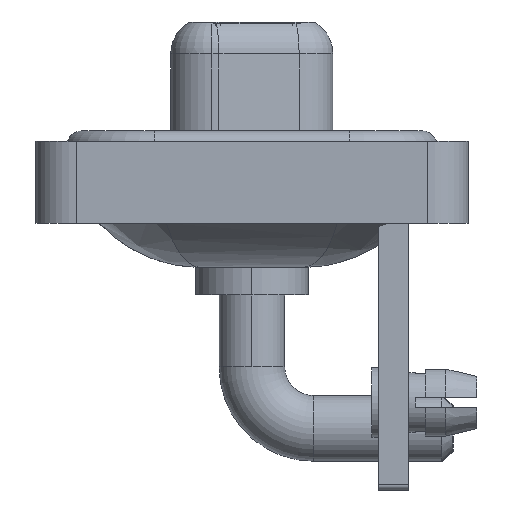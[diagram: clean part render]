
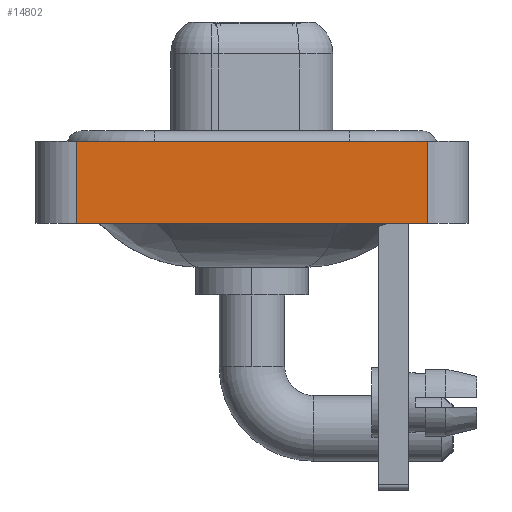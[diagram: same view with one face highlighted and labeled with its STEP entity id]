
A CAD part, left-side view. The second image highlights one B-rep face of the part: STEP entity #14802.
In plain terms, the highlighted planar face has unit normal (-1, 0, 0).
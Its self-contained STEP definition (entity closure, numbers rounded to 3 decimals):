
#95 = DIRECTION ( 'NONE',  ( 0., 0., 1. ) ) ;
#458 = ORIENTED_EDGE ( 'NONE', *, *, #13184, .T. ) ;
#964 = LINE ( 'NONE', #9850, #15194 ) ;
#982 = CARTESIAN_POINT ( 'NONE',  ( -7.25, 8.55, -3.6 ) ) ;
#1660 = CARTESIAN_POINT ( 'NONE',  ( -7.25, -8.55, -3.6 ) ) ;
#2927 = CARTESIAN_POINT ( 'NONE',  ( -7.25, -8.55, -3.6 ) ) ;
#3573 = LINE ( 'NONE', #8359, #3773 ) ;
#3686 = DIRECTION ( 'NONE',  ( -1., 0., 0. ) ) ;
#3773 = VECTOR ( 'NONE', #14341, 1000. ) ;
#4401 = VECTOR ( 'NONE', #17673, 1000. ) ;
#4481 = EDGE_CURVE ( 'NONE', #12451, #5096, #10329, .T. ) ;
#5096 = VERTEX_POINT ( 'NONE', #15277 ) ;
#5205 = EDGE_CURVE ( 'NONE', #12451, #12305, #9257, .T. ) ;
#6900 = ORIENTED_EDGE ( 'NONE', *, *, #12106, .F. ) ;
#7232 = CARTESIAN_POINT ( 'NONE',  ( -7.25, 8.55, -3.6 ) ) ;
#7726 = PLANE ( 'NONE',  #10907 ) ;
#8359 = CARTESIAN_POINT ( 'NONE',  ( -7.25, -8.55, 0.4 ) ) ;
#9175 = FACE_OUTER_BOUND ( 'NONE', #17970, .T. ) ;
#9257 = LINE ( 'NONE', #2927, #19062 ) ;
#9850 = CARTESIAN_POINT ( 'NONE',  ( -7.25, -8.55, -3.6 ) ) ;
#10329 = LINE ( 'NONE', #7232, #4401 ) ;
#10754 = CARTESIAN_POINT ( 'NONE',  ( -7.25, -8.55, -3.6 ) ) ;
#10907 = AXIS2_PLACEMENT_3D ( 'NONE', #1660, #3686, #95 ) ;
#12106 = EDGE_CURVE ( 'NONE', #5096, #14185, #3573, .T. ) ;
#12305 = VERTEX_POINT ( 'NONE', #10754 ) ;
#12451 = VERTEX_POINT ( 'NONE', #982 ) ;
#12696 = DIRECTION ( 'NONE',  ( 0., 0., 1. ) ) ;
#13150 = CARTESIAN_POINT ( 'NONE',  ( -7.25, -8.55, 0.4 ) ) ;
#13184 = EDGE_CURVE ( 'NONE', #12305, #14185, #964, .T. ) ;
#14185 = VERTEX_POINT ( 'NONE', #13150 ) ;
#14341 = DIRECTION ( 'NONE',  ( 0., -1., 0. ) ) ;
#14493 = ORIENTED_EDGE ( 'NONE', *, *, #5205, .T. ) ;
#14802 = ADVANCED_FACE ( 'NONE', ( #9175 ), #7726, .T. ) ;
#14857 = DIRECTION ( 'NONE',  ( 0., -1., 0. ) ) ;
#15194 = VECTOR ( 'NONE', #12696, 1000. ) ;
#15277 = CARTESIAN_POINT ( 'NONE',  ( -7.25, 8.55, 0.4 ) ) ;
#16851 = ORIENTED_EDGE ( 'NONE', *, *, #4481, .F. ) ;
#17673 = DIRECTION ( 'NONE',  ( 0., 0., 1. ) ) ;
#17970 = EDGE_LOOP ( 'NONE', ( #458, #6900, #16851, #14493 ) ) ;
#19062 = VECTOR ( 'NONE', #14857, 1000. ) ;
